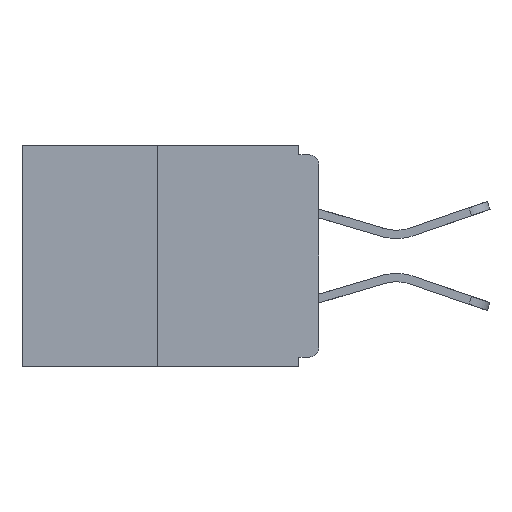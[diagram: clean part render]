
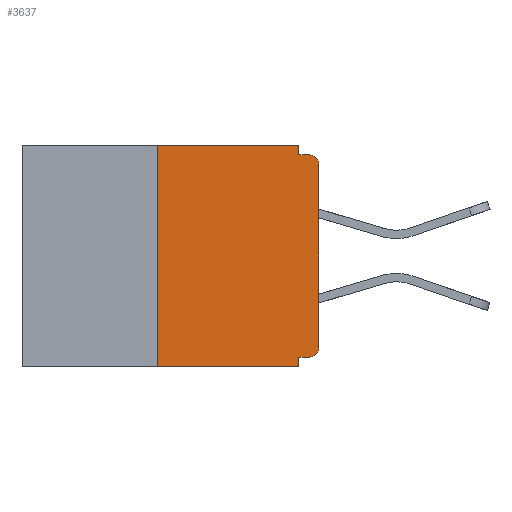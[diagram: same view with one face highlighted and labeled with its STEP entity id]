
A CAD part, left-side view. The second image highlights one B-rep face of the part: STEP entity #3637.
In plain terms, the highlighted planar face has unit normal (-1, 0, 0).
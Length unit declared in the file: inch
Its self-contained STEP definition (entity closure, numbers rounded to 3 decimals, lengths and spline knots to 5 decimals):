
#115 = DIRECTION ( 'NONE',  ( 0., 0., -1. ) ) ;
#151 = LINE ( 'NONE', #24197, #23327 ) ;
#274 = CARTESIAN_POINT ( 'NONE',  ( 0., 0.25, 0. ) ) ;
#1234 = VECTOR ( 'NONE', #2915, 39.37008 ) ;
#1809 = CARTESIAN_POINT ( 'NONE',  ( 0., 0.015, -0.313 ) ) ;
#1963 = VECTOR ( 'NONE', #17694, 39.37008 ) ;
#2237 = DIRECTION ( 'NONE',  ( -1., 0., 0. ) ) ;
#2285 = VECTOR ( 'NONE', #7971, 39.37008 ) ;
#2361 = DIRECTION ( 'NONE',  ( 0., -1., 0. ) ) ;
#2608 = PLANE ( 'NONE',  #25184 ) ;
#2915 = DIRECTION ( 'NONE',  ( 0., -1., 0. ) ) ;
#3336 = DIRECTION ( 'NONE',  ( 0., 0., -1. ) ) ;
#3428 = CARTESIAN_POINT ( 'NONE',  ( 0., 0.015, -0.015 ) ) ;
#3599 = EDGE_CURVE ( 'NONE', #8311, #25862, #23671, .T. ) ;
#3637 = ADVANCED_FACE ( 'NONE', ( #17245 ), #2608, .F. ) ;
#4202 = ORIENTED_EDGE ( 'NONE', *, *, #24447, .T. ) ;
#4595 = EDGE_CURVE ( 'NONE', #20297, #4761, #17567, .T. ) ;
#4761 = VERTEX_POINT ( 'NONE', #9832 ) ;
#4845 = ORIENTED_EDGE ( 'NONE', *, *, #4595, .F. ) ;
#5605 = ORIENTED_EDGE ( 'NONE', *, *, #12561, .F. ) ;
#5663 = ORIENTED_EDGE ( 'NONE', *, *, #26669, .F. ) ;
#5888 = CARTESIAN_POINT ( 'NONE',  ( 0., 0.46, 0. ) ) ;
#6339 = EDGE_CURVE ( 'NONE', #19731, #23416, #29872, .T. ) ;
#7187 = DIRECTION ( 'NONE',  ( 0., 0., -1. ) ) ;
#7316 = CARTESIAN_POINT ( 'NONE',  ( 0., 0., -0.328 ) ) ;
#7971 = DIRECTION ( 'NONE',  ( 0., 0., -1. ) ) ;
#8055 = ORIENTED_EDGE ( 'NONE', *, *, #24413, .T. ) ;
#8079 = CARTESIAN_POINT ( 'NONE',  ( 0., 0.031, -0.343 ) ) ;
#8311 = VERTEX_POINT ( 'NONE', #17804 ) ;
#9697 = DIRECTION ( 'NONE',  ( 0., 1., 0. ) ) ;
#9832 = CARTESIAN_POINT ( 'NONE',  ( 0., 0.031, -0.343 ) ) ;
#11465 = DIRECTION ( 'NONE',  ( 0., 0., -1. ) ) ;
#11766 = AXIS2_PLACEMENT_3D ( 'NONE', #30858, #2237, #3336 ) ;
#12089 = DIRECTION ( 'NONE',  ( 0., 0., 1. ) ) ;
#12200 = VERTEX_POINT ( 'NONE', #17895 ) ;
#12561 = EDGE_CURVE ( 'NONE', #12200, #17663, #30042, .T. ) ;
#12744 = VERTEX_POINT ( 'NONE', #26860 ) ;
#13147 = DIRECTION ( 'NONE',  ( 0., 0., 1. ) ) ;
#14108 = AXIS2_PLACEMENT_3D ( 'NONE', #1809, #28244, #11465 ) ;
#14219 = VECTOR ( 'NONE', #9697, 39.37008 ) ;
#14677 = VECTOR ( 'NONE', #12089, 39.37008 ) ;
#14958 = LINE ( 'NONE', #7316, #14219 ) ;
#15260 = LINE ( 'NONE', #27714, #24307 ) ;
#15645 = EDGE_CURVE ( 'NONE', #12200, #4761, #151, .T. ) ;
#16021 = CARTESIAN_POINT ( 'NONE',  ( 0., 0.031, -0.015 ) ) ;
#16452 = EDGE_CURVE ( 'NONE', #25862, #23416, #29241, .T. ) ;
#17245 = FACE_OUTER_BOUND ( 'NONE', #29562, .T. ) ;
#17567 = LINE ( 'NONE', #8079, #2285 ) ;
#17663 = VERTEX_POINT ( 'NONE', #29931 ) ;
#17694 = DIRECTION ( 'NONE',  ( 0., -1., 0. ) ) ;
#17804 = CARTESIAN_POINT ( 'NONE',  ( 0., 0.031, 0. ) ) ;
#17895 = CARTESIAN_POINT ( 'NONE',  ( 0., 0.25, -0.343 ) ) ;
#19468 = ORIENTED_EDGE ( 'NONE', *, *, #15645, .T. ) ;
#19513 = VECTOR ( 'NONE', #115, 39.37008 ) ;
#19731 = VERTEX_POINT ( 'NONE', #20755 ) ;
#20209 = ORIENTED_EDGE ( 'NONE', *, *, #3599, .F. ) ;
#20297 = VERTEX_POINT ( 'NONE', #29297 ) ;
#20407 = ORIENTED_EDGE ( 'NONE', *, *, #6339, .T. ) ;
#20755 = CARTESIAN_POINT ( 'NONE',  ( 0., 0., -0.03 ) ) ;
#21041 = LINE ( 'NONE', #5888, #1963 ) ;
#21534 = DIRECTION ( 'NONE',  ( 1., 0., 0. ) ) ;
#21727 = CARTESIAN_POINT ( 'NONE',  ( 0., 0.46, 0. ) ) ;
#22239 = CARTESIAN_POINT ( 'NONE',  ( 0., 0., -0.015 ) ) ;
#22699 = EDGE_CURVE ( 'NONE', #17663, #8311, #21041, .T. ) ;
#23327 = VECTOR ( 'NONE', #2361, 39.37008 ) ;
#23416 = VERTEX_POINT ( 'NONE', #3428 ) ;
#23671 = LINE ( 'NONE', #24258, #19513 ) ;
#24197 = CARTESIAN_POINT ( 'NONE',  ( 0., 0.46, -0.343 ) ) ;
#24258 = CARTESIAN_POINT ( 'NONE',  ( 0., 0.031, 0. ) ) ;
#24307 = VECTOR ( 'NONE', #13147, 39.37008 ) ;
#24413 = EDGE_CURVE ( 'NONE', #30600, #19731, #15260, .T. ) ;
#24447 = EDGE_CURVE ( 'NONE', #12744, #30600, #26162, .T. ) ;
#25184 = AXIS2_PLACEMENT_3D ( 'NONE', #21727, #21534, #7187 ) ;
#25862 = VERTEX_POINT ( 'NONE', #16021 ) ;
#26162 = CIRCLE ( 'NONE', #14108, 0.015 ) ;
#26565 = CARTESIAN_POINT ( 'NONE',  ( 0., 0., -0.313 ) ) ;
#26669 = EDGE_CURVE ( 'NONE', #12744, #20297, #14958, .T. ) ;
#26860 = CARTESIAN_POINT ( 'NONE',  ( 0., 0.015, -0.328 ) ) ;
#27148 = ORIENTED_EDGE ( 'NONE', *, *, #22699, .F. ) ;
#27714 = CARTESIAN_POINT ( 'NONE',  ( 0., 0., 0. ) ) ;
#28244 = DIRECTION ( 'NONE',  ( -1., 0., 0. ) ) ;
#29241 = LINE ( 'NONE', #22239, #1234 ) ;
#29297 = CARTESIAN_POINT ( 'NONE',  ( 0., 0.031, -0.328 ) ) ;
#29562 = EDGE_LOOP ( 'NONE', ( #27148, #5605, #19468, #4845, #5663, #4202, #8055, #20407, #30164, #20209 ) ) ;
#29872 = CIRCLE ( 'NONE', #11766, 0.015 ) ;
#29931 = CARTESIAN_POINT ( 'NONE',  ( 0., 0.25, 0. ) ) ;
#30042 = LINE ( 'NONE', #274, #14677 ) ;
#30164 = ORIENTED_EDGE ( 'NONE', *, *, #16452, .F. ) ;
#30600 = VERTEX_POINT ( 'NONE', #26565 ) ;
#30858 = CARTESIAN_POINT ( 'NONE',  ( 0., 0.015, -0.03 ) ) ;
